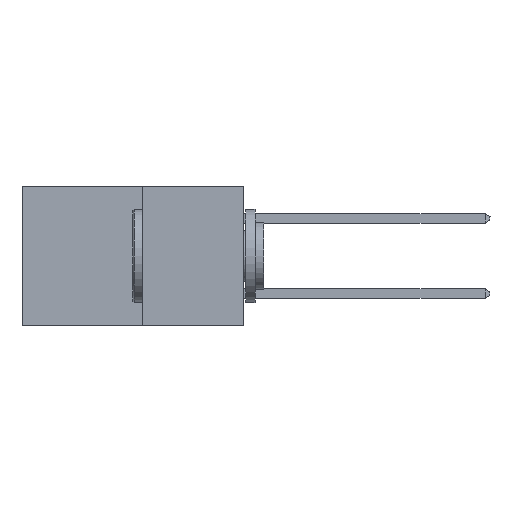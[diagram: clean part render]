
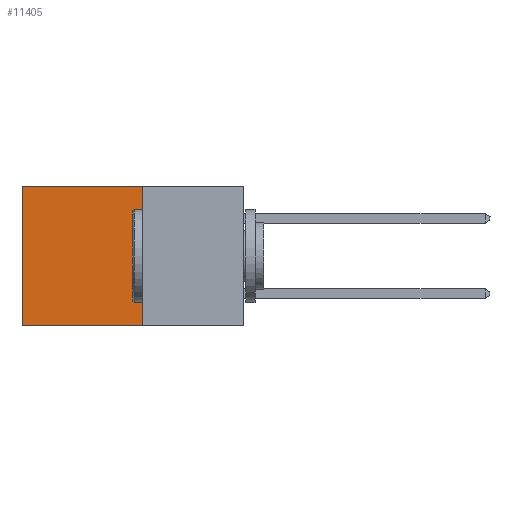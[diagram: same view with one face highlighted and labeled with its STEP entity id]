
A CAD part, left-side view. The second image highlights one B-rep face of the part: STEP entity #11405.
In plain terms, the highlighted planar face has unit normal (-1, 0, 0).
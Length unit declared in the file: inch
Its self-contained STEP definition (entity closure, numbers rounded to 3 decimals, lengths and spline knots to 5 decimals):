
#861 = LINE ( 'NONE', #28159, #25364 ) ;
#2147 = DIRECTION ( 'NONE',  ( 0., 1., 0. ) ) ;
#2154 = LINE ( 'NONE', #12844, #7738 ) ;
#3432 = VERTEX_POINT ( 'NONE', #15437 ) ;
#3672 = CARTESIAN_POINT ( 'NONE',  ( 0.277, 0.59, 0. ) ) ;
#5264 = DIRECTION ( 'NONE',  ( 1., 0., 0. ) ) ;
#5285 = ORIENTED_EDGE ( 'NONE', *, *, #19102, .F. ) ;
#7738 = VECTOR ( 'NONE', #27179, 39.37008 ) ;
#7802 = ORIENTED_EDGE ( 'NONE', *, *, #27846, .F. ) ;
#8102 = VERTEX_POINT ( 'NONE', #12672 ) ;
#8599 = CARTESIAN_POINT ( 'NONE',  ( 0.277, 0.27, 0. ) ) ;
#8882 = EDGE_CURVE ( 'NONE', #26430, #3432, #2154, .T. ) ;
#10316 = VECTOR ( 'NONE', #10961, 39.37008 ) ;
#10545 = VERTEX_POINT ( 'NONE', #21267 ) ;
#10961 = DIRECTION ( 'NONE',  ( 0., 1., 0. ) ) ;
#11405 = ADVANCED_FACE ( 'NONE', ( #21890 ), #26597, .F. ) ;
#12672 = CARTESIAN_POINT ( 'NONE',  ( 0.277, 0.27, 0. ) ) ;
#12810 = AXIS2_PLACEMENT_3D ( 'NONE', #24251, #5264, #28972 ) ;
#12844 = CARTESIAN_POINT ( 'NONE',  ( 0.277, 0.59, -0.37 ) ) ;
#14626 = LINE ( 'NONE', #15064, #26478 ) ;
#14815 = ORIENTED_EDGE ( 'NONE', *, *, #8882, .T. ) ;
#15064 = CARTESIAN_POINT ( 'NONE',  ( 0.277, 0.27, -0.37 ) ) ;
#15437 = CARTESIAN_POINT ( 'NONE',  ( 0.277, 0.59, -0.37 ) ) ;
#19102 = EDGE_CURVE ( 'NONE', #10545, #3432, #861, .T. ) ;
#19214 = EDGE_LOOP ( 'NONE', ( #14815, #5285, #7802, #22570 ) ) ;
#19820 = DIRECTION ( 'NONE',  ( 0., 0., -1. ) ) ;
#21267 = CARTESIAN_POINT ( 'NONE',  ( 0.277, 0.27, -0.37 ) ) ;
#21890 = FACE_OUTER_BOUND ( 'NONE', #19214, .T. ) ;
#22570 = ORIENTED_EDGE ( 'NONE', *, *, #29891, .T. ) ;
#24251 = CARTESIAN_POINT ( 'NONE',  ( 0.277, 0.27, -0.37 ) ) ;
#25364 = VECTOR ( 'NONE', #2147, 39.37008 ) ;
#26430 = VERTEX_POINT ( 'NONE', #3672 ) ;
#26478 = VECTOR ( 'NONE', #19820, 39.37008 ) ;
#26597 = PLANE ( 'NONE',  #12810 ) ;
#27179 = DIRECTION ( 'NONE',  ( 0., 0., -1. ) ) ;
#27846 = EDGE_CURVE ( 'NONE', #8102, #10545, #14626, .T. ) ;
#28159 = CARTESIAN_POINT ( 'NONE',  ( 0.277, 0.27, -0.37 ) ) ;
#28972 = DIRECTION ( 'NONE',  ( 0., 0., -1. ) ) ;
#29205 = LINE ( 'NONE', #8599, #10316 ) ;
#29891 = EDGE_CURVE ( 'NONE', #8102, #26430, #29205, .T. ) ;
